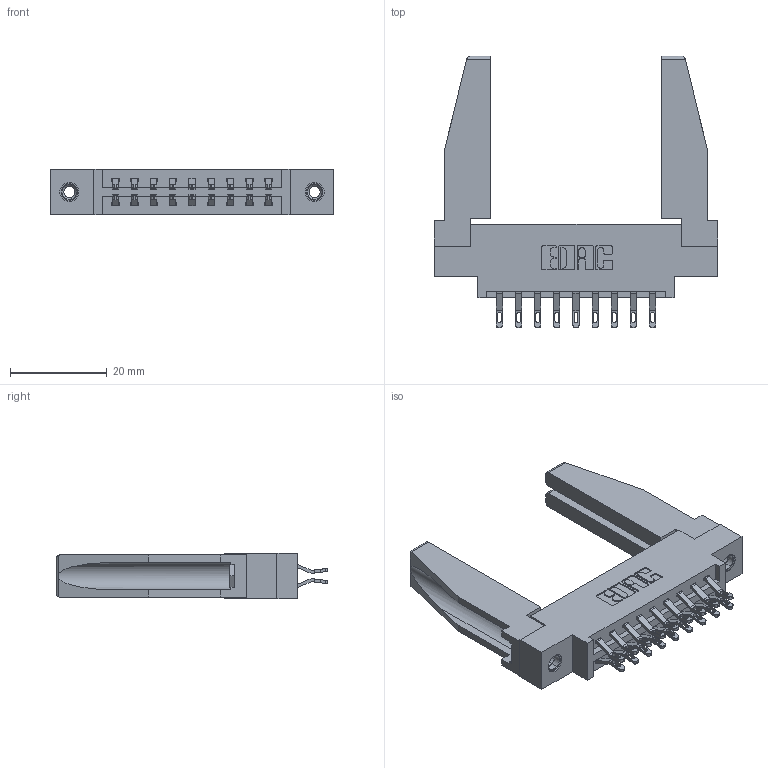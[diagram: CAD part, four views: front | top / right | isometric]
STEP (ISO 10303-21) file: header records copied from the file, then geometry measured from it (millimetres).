
FILE_DESCRIPTION (( 'STEP AP203' ), '1' );
FILE_NAME ('337-018-555-878.STEP', '2019-10-10T18:54:09', ( '' ), ( '' ), 'SwSTEP 2.0', 'SolidWorks 2016', '' );
FILE_SCHEMA (( 'CONFIG_CONTROL_DESIGN' ));
Length unit declared in the file: inch
Products named in the file (5): 345-292-001_555 Tail; 307-220-078; 337 Part_0.170 Offset - 0.156 Dia-TI; 337-018-555-878; 345-250-001_345-250-001-102
Assembly tree (23 placements, depth 2):
  337-018-555-878
    337 Part_0.170 Offset - 0.156 Dia-TI
    345-292-001_555 Tail  x18
    345-250-001_345-250-001-102  x2
    307-220-078  x2
Bounding box: 58.67 x 56.27 x 9.4 mm (x, y, z)
Volume: 9672.3 mm3; surface area: 10234.6 mm2
Topology: 23 solids, 23 shells, 1328 faces, 4055 edges, 2694 vertices
Faces by surface type: plane 806, cylinder 506, cone 12, torus 4
Entity records: 14144 total; most frequent: CARTESIAN_POINT 2446, ORIENTED_EDGE 2308, DIRECTION 2118, EDGE_CURVE 1154, VECTOR 968, LINE 968, VERTEX_POINT 764, AXIS2_PLACEMENT_3D 575
